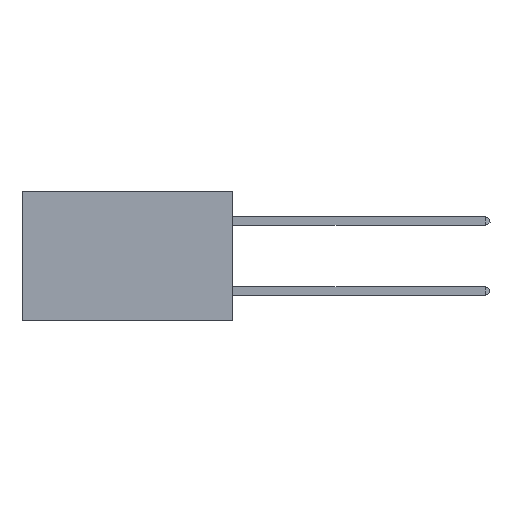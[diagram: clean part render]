
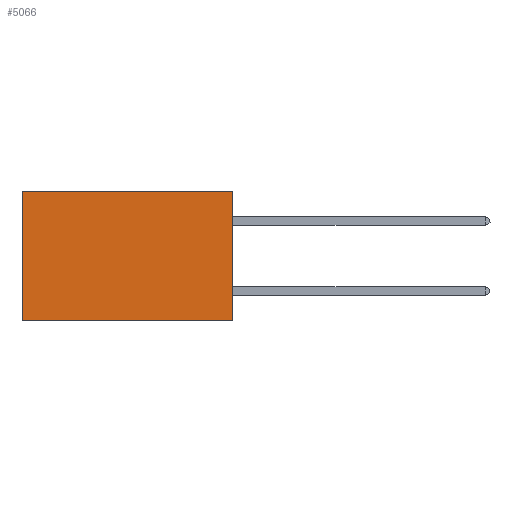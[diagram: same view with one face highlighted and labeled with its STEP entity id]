
A CAD part, left-side view. The second image highlights one B-rep face of the part: STEP entity #5066.
In plain terms, the highlighted planar face has unit normal (-1, 0, 0).
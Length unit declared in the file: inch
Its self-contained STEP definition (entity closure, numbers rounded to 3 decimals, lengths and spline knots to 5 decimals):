
#594 = LINE ( 'NONE', #2161, #17376 ) ;
#784 = VERTEX_POINT ( 'NONE', #15345 ) ;
#1048 = CARTESIAN_POINT ( 'NONE',  ( 0.2875, 0., -0.37 ) ) ;
#1758 = CARTESIAN_POINT ( 'NONE',  ( 0.2875, 0., -0.37 ) ) ;
#2161 = CARTESIAN_POINT ( 'NONE',  ( 0.2875, 0., 0. ) ) ;
#2681 = CARTESIAN_POINT ( 'NONE',  ( 0.2875, 0.6, 0. ) ) ;
#3496 = EDGE_LOOP ( 'NONE', ( #16895, #13057, #14813, #6860 ) ) ;
#3501 = VECTOR ( 'NONE', #15871, 39.37008 ) ;
#4812 = PLANE ( 'NONE',  #5289 ) ;
#5066 = ADVANCED_FACE ( 'NONE', ( #10580 ), #4812, .F. ) ;
#5074 = EDGE_CURVE ( 'NONE', #10622, #15669, #594, .T. ) ;
#5289 = AXIS2_PLACEMENT_3D ( 'NONE', #10320, #15672, #14360 ) ;
#5367 = DIRECTION ( 'NONE',  ( 0., 1., 0. ) ) ;
#5756 = EDGE_CURVE ( 'NONE', #11810, #784, #11197, .T. ) ;
#5998 = VECTOR ( 'NONE', #5367, 39.37008 ) ;
#6860 = ORIENTED_EDGE ( 'NONE', *, *, #7820, .T. ) ;
#7820 = EDGE_CURVE ( 'NONE', #10622, #11810, #8753, .T. ) ;
#8753 = LINE ( 'NONE', #10758, #5998 ) ;
#10320 = CARTESIAN_POINT ( 'NONE',  ( 0.2875, 0., 0. ) ) ;
#10580 = FACE_OUTER_BOUND ( 'NONE', #3496, .T. ) ;
#10622 = VERTEX_POINT ( 'NONE', #12170 ) ;
#10758 = CARTESIAN_POINT ( 'NONE',  ( 0.2875, 0., 0. ) ) ;
#11197 = LINE ( 'NONE', #11961, #3501 ) ;
#11643 = DIRECTION ( 'NONE',  ( 0., 0., -1. ) ) ;
#11810 = VERTEX_POINT ( 'NONE', #2681 ) ;
#11961 = CARTESIAN_POINT ( 'NONE',  ( 0.2875, 0.6, 0. ) ) ;
#11966 = EDGE_CURVE ( 'NONE', #15669, #784, #12286, .T. ) ;
#12170 = CARTESIAN_POINT ( 'NONE',  ( 0.2875, 0., 0. ) ) ;
#12286 = LINE ( 'NONE', #1758, #17163 ) ;
#13057 = ORIENTED_EDGE ( 'NONE', *, *, #11966, .F. ) ;
#13752 = DIRECTION ( 'NONE',  ( 0., 1., 0. ) ) ;
#14360 = DIRECTION ( 'NONE',  ( 0., 0., -1. ) ) ;
#14813 = ORIENTED_EDGE ( 'NONE', *, *, #5074, .F. ) ;
#15345 = CARTESIAN_POINT ( 'NONE',  ( 0.2875, 0.6, -0.37 ) ) ;
#15669 = VERTEX_POINT ( 'NONE', #1048 ) ;
#15672 = DIRECTION ( 'NONE',  ( 1., 0., 0. ) ) ;
#15871 = DIRECTION ( 'NONE',  ( 0., 0., -1. ) ) ;
#16895 = ORIENTED_EDGE ( 'NONE', *, *, #5756, .T. ) ;
#17163 = VECTOR ( 'NONE', #13752, 39.37008 ) ;
#17376 = VECTOR ( 'NONE', #11643, 39.37008 ) ;
